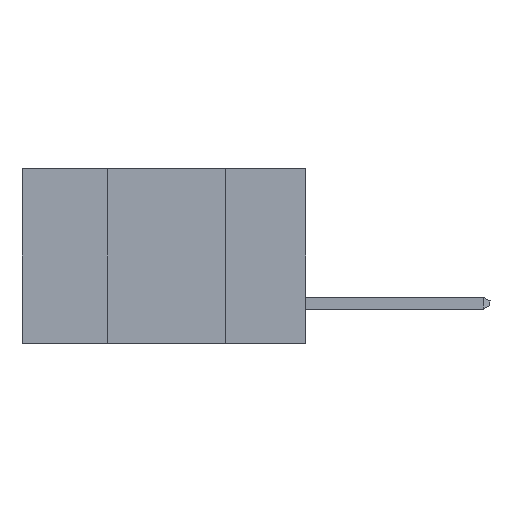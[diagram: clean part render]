
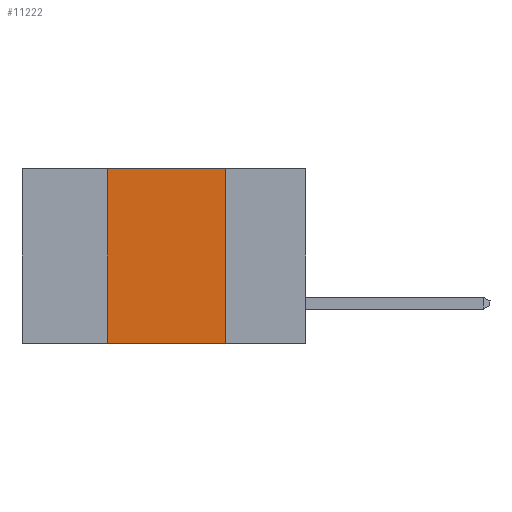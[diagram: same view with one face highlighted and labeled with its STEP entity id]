
A CAD part, left-side view. The second image highlights one B-rep face of the part: STEP entity #11222.
In plain terms, the highlighted planar face has unit normal (-1, 0, 0).
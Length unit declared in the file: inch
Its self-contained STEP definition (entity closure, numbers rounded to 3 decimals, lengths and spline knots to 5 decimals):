
#727 = VECTOR ( 'NONE', #13511, 39.37008 ) ;
#1008 = CARTESIAN_POINT ( 'NONE',  ( 0., 0.6, 0. ) ) ;
#2022 = LINE ( 'NONE', #6880, #2556 ) ;
#2122 = EDGE_CURVE ( 'NONE', #5578, #4781, #2022, .T. ) ;
#2158 = EDGE_CURVE ( 'NONE', #5952, #4781, #7441, .T. ) ;
#2556 = VECTOR ( 'NONE', #8027, 39.37008 ) ;
#2977 = VECTOR ( 'NONE', #14528, 39.37008 ) ;
#3017 = AXIS2_PLACEMENT_3D ( 'NONE', #6441, #15204, #10469 ) ;
#3484 = ORIENTED_EDGE ( 'NONE', *, *, #2122, .T. ) ;
#3701 = ORIENTED_EDGE ( 'NONE', *, *, #4395, .F. ) ;
#3858 = LINE ( 'NONE', #4923, #6923 ) ;
#4395 = EDGE_CURVE ( 'NONE', #15707, #5952, #11186, .T. ) ;
#4781 = VERTEX_POINT ( 'NONE', #8452 ) ;
#4923 = CARTESIAN_POINT ( 'NONE',  ( 0., 0.42, -0.37 ) ) ;
#5365 = PLANE ( 'NONE',  #3017 ) ;
#5578 = VERTEX_POINT ( 'NONE', #15193 ) ;
#5931 = ORIENTED_EDGE ( 'NONE', *, *, #11561, .F. ) ;
#5952 = VERTEX_POINT ( 'NONE', #10088 ) ;
#6441 = CARTESIAN_POINT ( 'NONE',  ( 0., 0.6, 0. ) ) ;
#6880 = CARTESIAN_POINT ( 'NONE',  ( 0., 0.6, -0.37 ) ) ;
#6923 = VECTOR ( 'NONE', #15223, 39.37008 ) ;
#7441 = LINE ( 'NONE', #12439, #727 ) ;
#8027 = DIRECTION ( 'NONE',  ( 0., -1., 0. ) ) ;
#8121 = CARTESIAN_POINT ( 'NONE',  ( 0., 0.42, 0. ) ) ;
#8452 = CARTESIAN_POINT ( 'NONE',  ( 0., 0.17, -0.37 ) ) ;
#8583 = ORIENTED_EDGE ( 'NONE', *, *, #2158, .F. ) ;
#10088 = CARTESIAN_POINT ( 'NONE',  ( 0., 0.17, 0. ) ) ;
#10469 = DIRECTION ( 'NONE',  ( 0., 0., -1. ) ) ;
#10538 = FACE_OUTER_BOUND ( 'NONE', #11292, .T. ) ;
#11186 = LINE ( 'NONE', #1008, #2977 ) ;
#11222 = ADVANCED_FACE ( 'NONE', ( #10538 ), #5365, .F. ) ;
#11292 = EDGE_LOOP ( 'NONE', ( #8583, #3701, #5931, #3484 ) ) ;
#11561 = EDGE_CURVE ( 'NONE', #5578, #15707, #3858, .T. ) ;
#12439 = CARTESIAN_POINT ( 'NONE',  ( 0., 0.17, -0.37 ) ) ;
#13511 = DIRECTION ( 'NONE',  ( 0., 0., -1. ) ) ;
#14528 = DIRECTION ( 'NONE',  ( 0., -1., 0. ) ) ;
#15193 = CARTESIAN_POINT ( 'NONE',  ( 0., 0.42, -0.37 ) ) ;
#15204 = DIRECTION ( 'NONE',  ( 1., 0., 0. ) ) ;
#15223 = DIRECTION ( 'NONE',  ( 0., 0., 1. ) ) ;
#15707 = VERTEX_POINT ( 'NONE', #8121 ) ;
